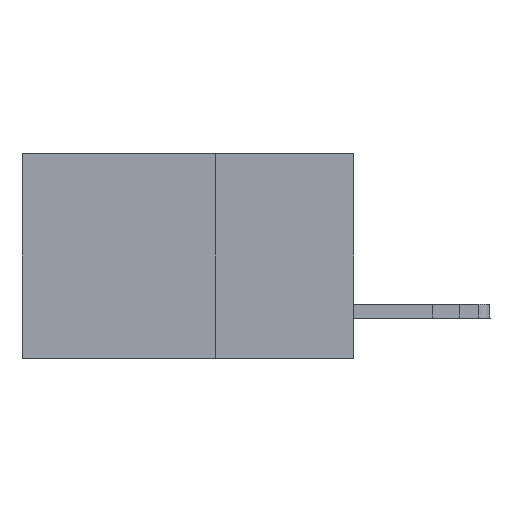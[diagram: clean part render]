
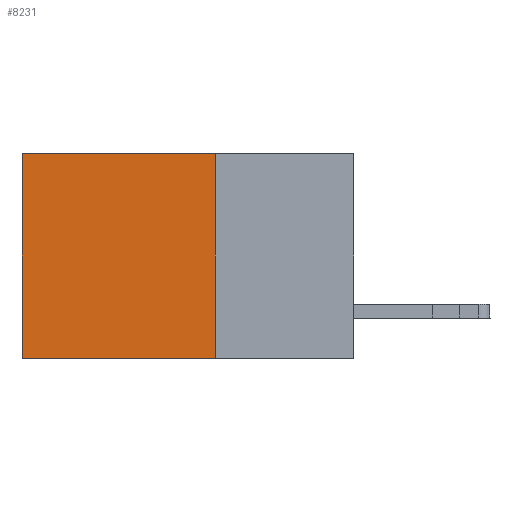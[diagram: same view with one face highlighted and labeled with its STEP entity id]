
A CAD part, left-side view. The second image highlights one B-rep face of the part: STEP entity #8231.
In plain terms, the highlighted planar face has unit normal (-1, 0, 0).
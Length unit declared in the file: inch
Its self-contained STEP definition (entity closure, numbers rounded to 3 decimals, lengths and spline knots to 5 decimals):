
#229 = VECTOR ( 'NONE', #2159, 39.37008 ) ;
#320 = LINE ( 'NONE', #11588, #5853 ) ;
#730 = CARTESIAN_POINT ( 'NONE',  ( 0.2875, 0.6, 0. ) ) ;
#1418 = CARTESIAN_POINT ( 'NONE',  ( 0.2875, 0.6, 0. ) ) ;
#2001 = VERTEX_POINT ( 'NONE', #730 ) ;
#2159 = DIRECTION ( 'NONE',  ( 0., 1., 0. ) ) ;
#2479 = FACE_OUTER_BOUND ( 'NONE', #10386, .T. ) ;
#3843 = LINE ( 'NONE', #13786, #229 ) ;
#3973 = DIRECTION ( 'NONE',  ( 0., 0., -1. ) ) ;
#4054 = LINE ( 'NONE', #1418, #17935 ) ;
#4250 = LINE ( 'NONE', #17138, #18180 ) ;
#5070 = VERTEX_POINT ( 'NONE', #10067 ) ;
#5853 = VECTOR ( 'NONE', #10079, 39.37008 ) ;
#6990 = DIRECTION ( 'NONE',  ( 1., 0., 0. ) ) ;
#8231 = ADVANCED_FACE ( 'NONE', ( #2479 ), #11204, .F. ) ;
#8349 = EDGE_CURVE ( 'NONE', #11076, #5070, #320, .T. ) ;
#9878 = DIRECTION ( 'NONE',  ( 0., 1., 0. ) ) ;
#9978 = EDGE_CURVE ( 'NONE', #2001, #12256, #4054, .T. ) ;
#10067 = CARTESIAN_POINT ( 'NONE',  ( 0.2875, 0.25, -0.37 ) ) ;
#10079 = DIRECTION ( 'NONE',  ( 0., 0., -1. ) ) ;
#10386 = EDGE_LOOP ( 'NONE', ( #11068, #14088, #13309, #13896 ) ) ;
#11068 = ORIENTED_EDGE ( 'NONE', *, *, #9978, .T. ) ;
#11076 = VERTEX_POINT ( 'NONE', #13561 ) ;
#11204 = PLANE ( 'NONE',  #14199 ) ;
#11588 = CARTESIAN_POINT ( 'NONE',  ( 0.2875, 0.25, 0. ) ) ;
#12256 = VERTEX_POINT ( 'NONE', #15273 ) ;
#12798 = DIRECTION ( 'NONE',  ( 0., 0., -1. ) ) ;
#12812 = EDGE_CURVE ( 'NONE', #5070, #12256, #4250, .T. ) ;
#13309 = ORIENTED_EDGE ( 'NONE', *, *, #8349, .F. ) ;
#13561 = CARTESIAN_POINT ( 'NONE',  ( 0.2875, 0.25, 0. ) ) ;
#13786 = CARTESIAN_POINT ( 'NONE',  ( 0.2875, 0.25, 0. ) ) ;
#13896 = ORIENTED_EDGE ( 'NONE', *, *, #14870, .T. ) ;
#14088 = ORIENTED_EDGE ( 'NONE', *, *, #12812, .F. ) ;
#14199 = AXIS2_PLACEMENT_3D ( 'NONE', #17153, #6990, #12798 ) ;
#14870 = EDGE_CURVE ( 'NONE', #11076, #2001, #3843, .T. ) ;
#15273 = CARTESIAN_POINT ( 'NONE',  ( 0.2875, 0.6, -0.37 ) ) ;
#17138 = CARTESIAN_POINT ( 'NONE',  ( 0.2875, 0.25, -0.37 ) ) ;
#17153 = CARTESIAN_POINT ( 'NONE',  ( 0.2875, 0.25, 0. ) ) ;
#17935 = VECTOR ( 'NONE', #3973, 39.37008 ) ;
#18180 = VECTOR ( 'NONE', #9878, 39.37008 ) ;
